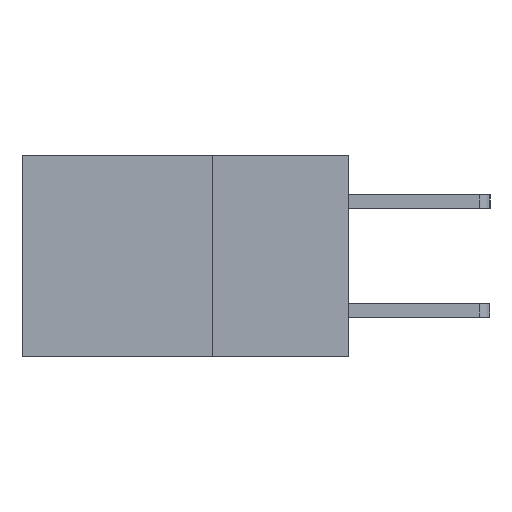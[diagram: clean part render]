
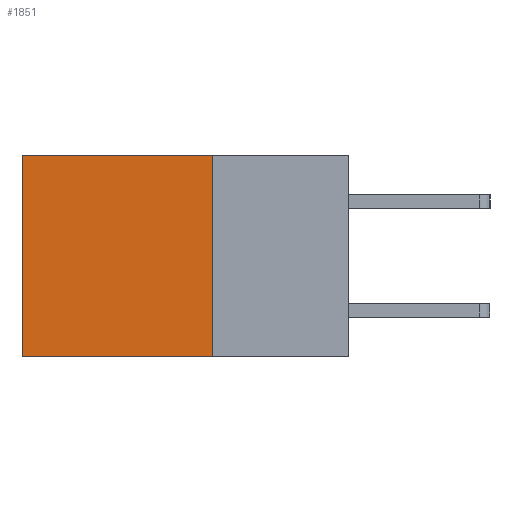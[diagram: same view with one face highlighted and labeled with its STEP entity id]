
A CAD part, left-side view. The second image highlights one B-rep face of the part: STEP entity #1851.
In plain terms, the highlighted planar face has unit normal (-1, 0, 0).
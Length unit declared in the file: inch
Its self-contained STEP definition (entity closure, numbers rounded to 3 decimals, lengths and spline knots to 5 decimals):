
#699 = CARTESIAN_POINT ( 'NONE',  ( 0.298, 0.6, -0.37 ) ) ;
#814 = PLANE ( 'NONE',  #7121 ) ;
#1098 = LINE ( 'NONE', #4372, #2934 ) ;
#1851 = ADVANCED_FACE ( 'NONE', ( #8244 ), #814, .F. ) ;
#1990 = LINE ( 'NONE', #9008, #2238 ) ;
#2134 = EDGE_CURVE ( 'NONE', #3585, #7761, #9796, .T. ) ;
#2238 = VECTOR ( 'NONE', #6102, 39.37008 ) ;
#2604 = EDGE_LOOP ( 'NONE', ( #7842, #5294, #3933, #8330 ) ) ;
#2934 = VECTOR ( 'NONE', #4134, 39.37008 ) ;
#3191 = CARTESIAN_POINT ( 'NONE',  ( 0.298, 0.25, 0. ) ) ;
#3395 = VERTEX_POINT ( 'NONE', #699 ) ;
#3585 = VERTEX_POINT ( 'NONE', #9431 ) ;
#3638 = CARTESIAN_POINT ( 'NONE',  ( 0.298, 0.25, -0.37 ) ) ;
#3668 = DIRECTION ( 'NONE',  ( 0., 1., 0. ) ) ;
#3735 = DIRECTION ( 'NONE',  ( 0., 1., 0. ) ) ;
#3796 = LINE ( 'NONE', #3638, #5598 ) ;
#3933 = ORIENTED_EDGE ( 'NONE', *, *, #8399, .F. ) ;
#4134 = DIRECTION ( 'NONE',  ( 0., 0., -1. ) ) ;
#4372 = CARTESIAN_POINT ( 'NONE',  ( 0.298, 0.6, 0. ) ) ;
#4655 = CARTESIAN_POINT ( 'NONE',  ( 0.298, 0.6, 0. ) ) ;
#4780 = VERTEX_POINT ( 'NONE', #6623 ) ;
#5294 = ORIENTED_EDGE ( 'NONE', *, *, #8037, .F. ) ;
#5410 = DIRECTION ( 'NONE',  ( 0., 0., -1. ) ) ;
#5598 = VECTOR ( 'NONE', #3668, 39.37008 ) ;
#6102 = DIRECTION ( 'NONE',  ( 0., 0., -1. ) ) ;
#6120 = VECTOR ( 'NONE', #3735, 39.37008 ) ;
#6623 = CARTESIAN_POINT ( 'NONE',  ( 0.298, 0.25, -0.37 ) ) ;
#7121 = AXIS2_PLACEMENT_3D ( 'NONE', #7583, #9345, #5410 ) ;
#7583 = CARTESIAN_POINT ( 'NONE',  ( 0.298, 0.25, 0. ) ) ;
#7761 = VERTEX_POINT ( 'NONE', #4655 ) ;
#7842 = ORIENTED_EDGE ( 'NONE', *, *, #9096, .T. ) ;
#8037 = EDGE_CURVE ( 'NONE', #4780, #3395, #3796, .T. ) ;
#8244 = FACE_OUTER_BOUND ( 'NONE', #2604, .T. ) ;
#8330 = ORIENTED_EDGE ( 'NONE', *, *, #2134, .T. ) ;
#8399 = EDGE_CURVE ( 'NONE', #3585, #4780, #1990, .T. ) ;
#9008 = CARTESIAN_POINT ( 'NONE',  ( 0.298, 0.25, 0. ) ) ;
#9096 = EDGE_CURVE ( 'NONE', #7761, #3395, #1098, .T. ) ;
#9345 = DIRECTION ( 'NONE',  ( 1., 0., 0. ) ) ;
#9431 = CARTESIAN_POINT ( 'NONE',  ( 0.298, 0.25, 0. ) ) ;
#9796 = LINE ( 'NONE', #3191, #6120 ) ;
